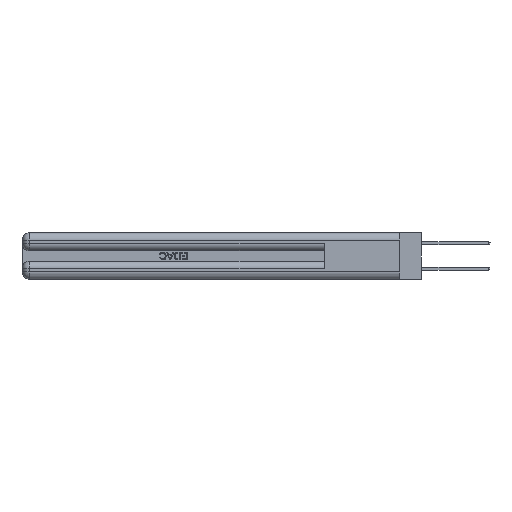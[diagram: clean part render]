
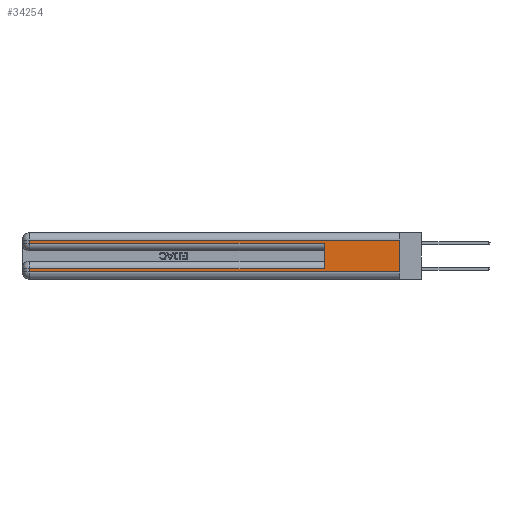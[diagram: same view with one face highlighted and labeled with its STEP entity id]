
A CAD part, left-side view. The second image highlights one B-rep face of the part: STEP entity #34254.
In plain terms, the highlighted planar face has unit normal (-1, 0, 0).
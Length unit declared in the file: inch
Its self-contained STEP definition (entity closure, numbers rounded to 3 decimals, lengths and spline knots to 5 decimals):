
#1854 = LINE ( 'NONE', #39681, #7929 ) ;
#1920 = LINE ( 'NONE', #30840, #49638 ) ;
#2251 = VERTEX_POINT ( 'NONE', #12109 ) ;
#2905 = ORIENTED_EDGE ( 'NONE', *, *, #30666, .T. ) ;
#3567 = LINE ( 'NONE', #18517, #10864 ) ;
#4703 = DIRECTION ( 'NONE',  ( 0., 0., -1. ) ) ;
#5416 = EDGE_LOOP ( 'NONE', ( #48893, #25642, #34748, #23182, #24564, #2905, #29512, #40948 ) ) ;
#6329 = EDGE_CURVE ( 'NONE', #27718, #45879, #36803, .T. ) ;
#7777 = CARTESIAN_POINT ( 'NONE',  ( 0., 0., 0.285 ) ) ;
#7929 = VECTOR ( 'NONE', #12878, 39.37008 ) ;
#8597 = CARTESIAN_POINT ( 'NONE',  ( 0., 0., 0.37 ) ) ;
#9011 = CARTESIAN_POINT ( 'NONE',  ( 0., 0., 0.37 ) ) ;
#9827 = LINE ( 'NONE', #16781, #21295 ) ;
#10864 = VECTOR ( 'NONE', #22438, 39.37008 ) ;
#11111 = EDGE_CURVE ( 'NONE', #25530, #45226, #43495, .T. ) ;
#11768 = LINE ( 'NONE', #24842, #33497 ) ;
#12109 = CARTESIAN_POINT ( 'NONE',  ( 0., 2.94, 0.085 ) ) ;
#12878 = DIRECTION ( 'NONE',  ( 0., -1., 0. ) ) ;
#13606 = CARTESIAN_POINT ( 'NONE',  ( 0., 2.94, 0.31 ) ) ;
#14925 = CARTESIAN_POINT ( 'NONE',  ( 0., 0.6, 0.285 ) ) ;
#15158 = EDGE_CURVE ( 'NONE', #2251, #43216, #11768, .T. ) ;
#15830 = VECTOR ( 'NONE', #19565, 39.37008 ) ;
#16632 = EDGE_CURVE ( 'NONE', #45366, #45879, #21850, .T. ) ;
#16781 = CARTESIAN_POINT ( 'NONE',  ( 0., 0., 0.085 ) ) ;
#17349 = DIRECTION ( 'NONE',  ( 0., 0., -1. ) ) ;
#18517 = CARTESIAN_POINT ( 'NONE',  ( 0., 0., 0.31 ) ) ;
#19565 = DIRECTION ( 'NONE',  ( 0., -1., 0. ) ) ;
#21005 = FACE_OUTER_BOUND ( 'NONE', #5416, .T. ) ;
#21238 = DIRECTION ( 'NONE',  ( 0., 0., 1. ) ) ;
#21295 = VECTOR ( 'NONE', #47334, 39.37008 ) ;
#21850 = LINE ( 'NONE', #7777, #15830 ) ;
#22438 = DIRECTION ( 'NONE',  ( 0., 1., 0. ) ) ;
#23182 = ORIENTED_EDGE ( 'NONE', *, *, #16632, .T. ) ;
#24564 = ORIENTED_EDGE ( 'NONE', *, *, #6329, .F. ) ;
#24842 = CARTESIAN_POINT ( 'NONE',  ( 0., 2.94, 0.37 ) ) ;
#25530 = VERTEX_POINT ( 'NONE', #25715 ) ;
#25642 = ORIENTED_EDGE ( 'NONE', *, *, #36590, .T. ) ;
#25715 = CARTESIAN_POINT ( 'NONE',  ( 0., 0., 0.31 ) ) ;
#25889 = DIRECTION ( 'NONE',  ( 0., 0., -1. ) ) ;
#27718 = VERTEX_POINT ( 'NONE', #41526 ) ;
#28707 = CARTESIAN_POINT ( 'NONE',  ( 0., 0.6, 0.145 ) ) ;
#29508 = CARTESIAN_POINT ( 'NONE',  ( 0., 0., 0.06 ) ) ;
#29512 = ORIENTED_EDGE ( 'NONE', *, *, #15158, .T. ) ;
#30666 = EDGE_CURVE ( 'NONE', #27718, #2251, #9827, .T. ) ;
#30840 = CARTESIAN_POINT ( 'NONE',  ( 0., 2.94, 0.37 ) ) ;
#31014 = DIRECTION ( 'NONE',  ( 0., 0., -1. ) ) ;
#31389 = EDGE_CURVE ( 'NONE', #43216, #45226, #1854, .T. ) ;
#32511 = CARTESIAN_POINT ( 'NONE',  ( 0., 2.94, 0.06 ) ) ;
#32615 = VECTOR ( 'NONE', #21238, 39.37008 ) ;
#33497 = VECTOR ( 'NONE', #17349, 39.37008 ) ;
#33964 = DIRECTION ( 'NONE',  ( 1., 0., 0. ) ) ;
#34204 = CARTESIAN_POINT ( 'NONE',  ( 0., 2.94, 0.285 ) ) ;
#34254 = ADVANCED_FACE ( 'NONE', ( #21005 ), #48803, .F. ) ;
#34748 = ORIENTED_EDGE ( 'NONE', *, *, #42953, .T. ) ;
#36590 = EDGE_CURVE ( 'NONE', #25530, #49035, #3567, .T. ) ;
#36803 = LINE ( 'NONE', #28707, #32615 ) ;
#38580 = AXIS2_PLACEMENT_3D ( 'NONE', #9011, #33964, #25889 ) ;
#39681 = CARTESIAN_POINT ( 'NONE',  ( 0., 0., 0.06 ) ) ;
#40948 = ORIENTED_EDGE ( 'NONE', *, *, #31389, .T. ) ;
#41526 = CARTESIAN_POINT ( 'NONE',  ( 0., 0.6, 0.085 ) ) ;
#42953 = EDGE_CURVE ( 'NONE', #49035, #45366, #1920, .T. ) ;
#43216 = VERTEX_POINT ( 'NONE', #32511 ) ;
#43495 = LINE ( 'NONE', #8597, #47123 ) ;
#45226 = VERTEX_POINT ( 'NONE', #29508 ) ;
#45366 = VERTEX_POINT ( 'NONE', #34204 ) ;
#45879 = VERTEX_POINT ( 'NONE', #14925 ) ;
#47123 = VECTOR ( 'NONE', #4703, 39.37008 ) ;
#47334 = DIRECTION ( 'NONE',  ( 0., 1., 0. ) ) ;
#48803 = PLANE ( 'NONE',  #38580 ) ;
#48893 = ORIENTED_EDGE ( 'NONE', *, *, #11111, .F. ) ;
#49035 = VERTEX_POINT ( 'NONE', #13606 ) ;
#49638 = VECTOR ( 'NONE', #31014, 39.37008 ) ;
